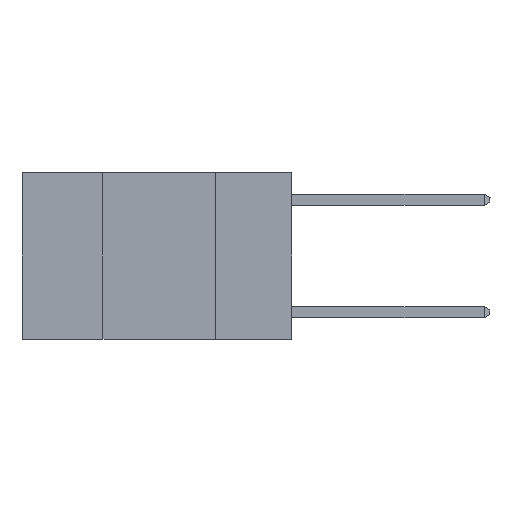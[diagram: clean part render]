
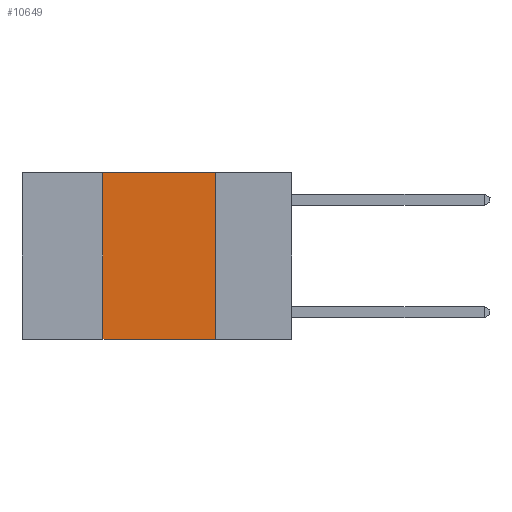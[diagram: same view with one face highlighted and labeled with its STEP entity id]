
A CAD part, left-side view. The second image highlights one B-rep face of the part: STEP entity #10649.
In plain terms, the highlighted planar face has unit normal (-1, 0, 0).
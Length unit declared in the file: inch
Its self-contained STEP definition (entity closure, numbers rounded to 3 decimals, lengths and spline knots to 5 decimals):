
#34 = LINE ( 'NONE', #5823, #8794 ) ;
#200 = DIRECTION ( 'NONE',  ( 0., 0., -1. ) ) ;
#210 = DIRECTION ( 'NONE',  ( 0., -1., 0. ) ) ;
#1623 = LINE ( 'NONE', #7781, #5696 ) ;
#2040 = VECTOR ( 'NONE', #210, 39.37008 ) ;
#3249 = VERTEX_POINT ( 'NONE', #17190 ) ;
#3727 = EDGE_CURVE ( 'NONE', #6640, #3249, #7699, .T. ) ;
#4195 = ORIENTED_EDGE ( 'NONE', *, *, #3727, .F. ) ;
#4204 = EDGE_CURVE ( 'NONE', #7419, #6825, #34, .T. ) ;
#5696 = VECTOR ( 'NONE', #13527, 39.37008 ) ;
#5823 = CARTESIAN_POINT ( 'NONE',  ( 0., 0.17, 0. ) ) ;
#5970 = ORIENTED_EDGE ( 'NONE', *, *, #6169, .F. ) ;
#6169 = EDGE_CURVE ( 'NONE', #3249, #7419, #11859, .T. ) ;
#6544 = CARTESIAN_POINT ( 'NONE',  ( 0., 0.6, 0. ) ) ;
#6586 = DIRECTION ( 'NONE',  ( 1., 0., 0. ) ) ;
#6640 = VERTEX_POINT ( 'NONE', #14742 ) ;
#6696 = ORIENTED_EDGE ( 'NONE', *, *, #4204, .F. ) ;
#6825 = VERTEX_POINT ( 'NONE', #15495 ) ;
#7419 = VERTEX_POINT ( 'NONE', #17817 ) ;
#7699 = LINE ( 'NONE', #16475, #12072 ) ;
#7781 = CARTESIAN_POINT ( 'NONE',  ( 0., 0.6, -0.37 ) ) ;
#7891 = EDGE_CURVE ( 'NONE', #6640, #6825, #1623, .T. ) ;
#8794 = VECTOR ( 'NONE', #200, 39.37008 ) ;
#10643 = CARTESIAN_POINT ( 'NONE',  ( 0., 0.6, 0. ) ) ;
#10649 = ADVANCED_FACE ( 'NONE', ( #12228 ), #18002, .F. ) ;
#11859 = LINE ( 'NONE', #6544, #2040 ) ;
#12072 = VECTOR ( 'NONE', #13437, 39.37008 ) ;
#12228 = FACE_OUTER_BOUND ( 'NONE', #14233, .T. ) ;
#13437 = DIRECTION ( 'NONE',  ( 0., 0., 1. ) ) ;
#13527 = DIRECTION ( 'NONE',  ( 0., -1., 0. ) ) ;
#14233 = EDGE_LOOP ( 'NONE', ( #6696, #5970, #4195, #16986 ) ) ;
#14742 = CARTESIAN_POINT ( 'NONE',  ( 0., 0.42, -0.37 ) ) ;
#14753 = AXIS2_PLACEMENT_3D ( 'NONE', #10643, #6586, #14900 ) ;
#14900 = DIRECTION ( 'NONE',  ( 0., 0., -1. ) ) ;
#15495 = CARTESIAN_POINT ( 'NONE',  ( 0., 0.17, -0.37 ) ) ;
#16475 = CARTESIAN_POINT ( 'NONE',  ( 0., 0.42, 0. ) ) ;
#16986 = ORIENTED_EDGE ( 'NONE', *, *, #7891, .T. ) ;
#17190 = CARTESIAN_POINT ( 'NONE',  ( 0., 0.42, 0. ) ) ;
#17817 = CARTESIAN_POINT ( 'NONE',  ( 0., 0.17, 0. ) ) ;
#18002 = PLANE ( 'NONE',  #14753 ) ;
